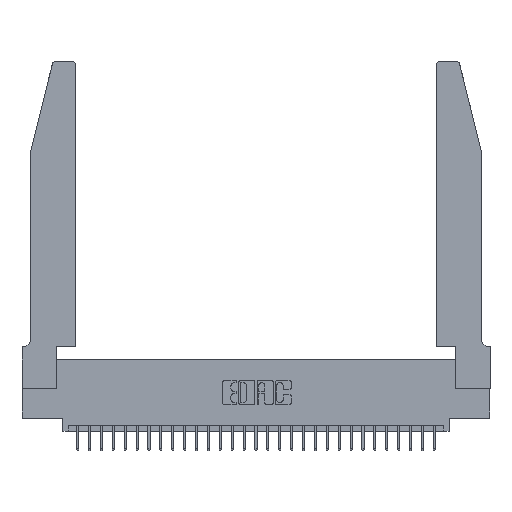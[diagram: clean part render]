
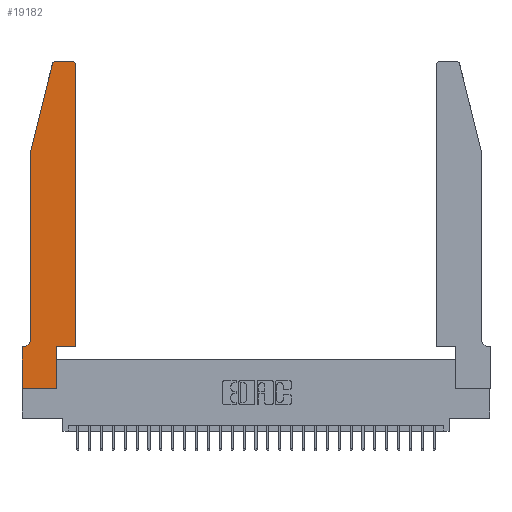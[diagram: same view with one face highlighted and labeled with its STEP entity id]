
A CAD part, top view. The second image highlights one B-rep face of the part: STEP entity #19182.
In plain terms, the highlighted planar face has unit normal (0, 0, 1).
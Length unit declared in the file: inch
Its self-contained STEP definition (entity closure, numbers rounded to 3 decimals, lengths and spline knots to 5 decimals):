
#178 = DIRECTION ( 'NONE',  ( 1., 0., 0. ) ) ;
#312 = LINE ( 'NONE', #15355, #5230 ) ;
#991 = ORIENTED_EDGE ( 'NONE', *, *, #17847, .T. ) ;
#1495 = CARTESIAN_POINT ( 'NONE',  ( 0.4505, 2.72, 0.37 ) ) ;
#1654 = CARTESIAN_POINT ( 'NONE',  ( 0.0755, 2., 0.37 ) ) ;
#1874 = CARTESIAN_POINT ( 'NONE',  ( 0.2865, 0.35, 0.37 ) ) ;
#2025 = VERTEX_POINT ( 'NONE', #1495 ) ;
#2200 = CARTESIAN_POINT ( 'NONE',  ( 0.284, 2.72, 0.37 ) ) ;
#2810 = CARTESIAN_POINT ( 'NONE',  ( 0.0755, 2., 0.37 ) ) ;
#3173 = VECTOR ( 'NONE', #6705, 39.37008 ) ;
#3685 = VECTOR ( 'NONE', #9991, 39.37008 ) ;
#4329 = ORIENTED_EDGE ( 'NONE', *, *, #30274, .T. ) ;
#4561 = CARTESIAN_POINT ( 'NONE',  ( 0.2865, 0.35, 0.37 ) ) ;
#4610 = DIRECTION ( 'NONE',  ( 1., 0., 0. ) ) ;
#4860 = VERTEX_POINT ( 'NONE', #24279 ) ;
#5037 = CARTESIAN_POINT ( 'NONE',  ( 0.4505, 0.35, 0.37 ) ) ;
#5230 = VECTOR ( 'NONE', #29594, 39.37008 ) ;
#6099 = LINE ( 'NONE', #14713, #30549 ) ;
#6434 = VECTOR ( 'NONE', #21768, 39.37008 ) ;
#6705 = DIRECTION ( 'NONE',  ( 0., 1., 0. ) ) ;
#7138 = DIRECTION ( 'NONE',  ( 0., 0., 1. ) ) ;
#7229 = VERTEX_POINT ( 'NONE', #8132 ) ;
#7371 = ORIENTED_EDGE ( 'NONE', *, *, #24773, .T. ) ;
#7495 = CARTESIAN_POINT ( 'NONE',  ( 0.2605, 2.75, 0.37 ) ) ;
#7584 = CARTESIAN_POINT ( 'NONE',  ( 0., 0., 0.37 ) ) ;
#7745 = EDGE_CURVE ( 'NONE', #14163, #13380, #26379, .T. ) ;
#7793 = CARTESIAN_POINT ( 'NONE',  ( 0., 0.35, 0.37 ) ) ;
#7902 = VECTOR ( 'NONE', #178, 39.37008 ) ;
#8132 = CARTESIAN_POINT ( 'NONE',  ( 0.0755, 2., 0.37 ) ) ;
#8502 = ORIENTED_EDGE ( 'NONE', *, *, #21854, .T. ) ;
#9805 = VERTEX_POINT ( 'NONE', #17820 ) ;
#9991 = DIRECTION ( 'NONE',  ( 1., 0., 0. ) ) ;
#10206 = DIRECTION ( 'NONE',  ( 1., 0., 0. ) ) ;
#10277 = LINE ( 'NONE', #1654, #28432 ) ;
#10327 = VERTEX_POINT ( 'NONE', #16941 ) ;
#10358 = EDGE_CURVE ( 'NONE', #25452, #18790, #20582, .T. ) ;
#10632 = DIRECTION ( 'NONE',  ( 0., 0., -1. ) ) ;
#10787 = LINE ( 'NONE', #7584, #3685 ) ;
#10956 = EDGE_CURVE ( 'NONE', #4860, #7229, #28655, .T. ) ;
#12542 = CARTESIAN_POINT ( 'NONE',  ( 0.2865, 0., 0.37 ) ) ;
#12802 = LINE ( 'NONE', #7495, #6434 ) ;
#13380 = VERTEX_POINT ( 'NONE', #18164 ) ;
#13464 = CARTESIAN_POINT ( 'NONE',  ( 0.4505, 0.35, 0.37 ) ) ;
#13768 = CIRCLE ( 'NONE', #21373, 0.03 ) ;
#14163 = VERTEX_POINT ( 'NONE', #16574 ) ;
#14263 = AXIS2_PLACEMENT_3D ( 'NONE', #24843, #10632, #27224 ) ;
#14713 = CARTESIAN_POINT ( 'NONE',  ( 0.0755, 0.35, 0.37 ) ) ;
#14776 = EDGE_CURVE ( 'NONE', #24351, #4860, #28100, .T. ) ;
#15027 = CARTESIAN_POINT ( 'NONE',  ( 0., 0.35, 0.37 ) ) ;
#15355 = CARTESIAN_POINT ( 'NONE',  ( 0., 0., 0.37 ) ) ;
#16107 = DIRECTION ( 'NONE',  ( 0., -1., 0. ) ) ;
#16574 = CARTESIAN_POINT ( 'NONE',  ( 0.0755, 0.42, 0.37 ) ) ;
#16941 = CARTESIAN_POINT ( 'NONE',  ( 0., 0., 0.37 ) ) ;
#17098 = DIRECTION ( 'NONE',  ( -1., 0., 0. ) ) ;
#17359 = EDGE_CURVE ( 'NONE', #30369, #10327, #312, .T. ) ;
#17457 = ORIENTED_EDGE ( 'NONE', *, *, #7745, .T. ) ;
#17577 = CARTESIAN_POINT ( 'NONE',  ( 0.4505, 0.35, 0.37 ) ) ;
#17629 = VECTOR ( 'NONE', #24807, 39.37008 ) ;
#17820 = CARTESIAN_POINT ( 'NONE',  ( 0.4205, 2.75, 0.37 ) ) ;
#17847 = EDGE_CURVE ( 'NONE', #10327, #26943, #10787, .T. ) ;
#18084 = EDGE_LOOP ( 'NONE', ( #4329, #27038, #27406, #7371, #17457, #28899, #24124, #991, #27813, #29283, #24515, #8502 ) ) ;
#18164 = CARTESIAN_POINT ( 'NONE',  ( 0.0055, 0.35, 0.37 ) ) ;
#18790 = VERTEX_POINT ( 'NONE', #13464 ) ;
#18932 = DIRECTION ( 'NONE',  ( 0., 0., 1. ) ) ;
#19182 = ADVANCED_FACE ( 'NONE', ( #20389 ), #24129, .T. ) ;
#19776 = AXIS2_PLACEMENT_3D ( 'NONE', #7793, #24444, #10206 ) ;
#20389 = FACE_OUTER_BOUND ( 'NONE', #18084, .T. ) ;
#20582 = LINE ( 'NONE', #5037, #7902 ) ;
#20944 = AXIS2_PLACEMENT_3D ( 'NONE', #2200, #18932, #4610 ) ;
#21373 = AXIS2_PLACEMENT_3D ( 'NONE', #21400, #7138, #23750 ) ;
#21400 = CARTESIAN_POINT ( 'NONE',  ( 0.4205, 2.72, 0.37 ) ) ;
#21768 = DIRECTION ( 'NONE',  ( -1., 0., 0. ) ) ;
#21854 = EDGE_CURVE ( 'NONE', #2025, #9805, #13768, .T. ) ;
#22399 = VECTOR ( 'NONE', #24263, 39.37008 ) ;
#23645 = LINE ( 'NONE', #1874, #3173 ) ;
#23750 = DIRECTION ( 'NONE',  ( 1., 0., 0. ) ) ;
#24124 = ORIENTED_EDGE ( 'NONE', *, *, #17359, .T. ) ;
#24129 = PLANE ( 'NONE',  #19776 ) ;
#24263 = DIRECTION ( 'NONE',  ( -0.239, -0.971, 0. ) ) ;
#24279 = CARTESIAN_POINT ( 'NONE',  ( 0.25487, 2.72718, 0.37 ) ) ;
#24351 = VERTEX_POINT ( 'NONE', #27957 ) ;
#24444 = DIRECTION ( 'NONE',  ( 0., 0., 1. ) ) ;
#24515 = ORIENTED_EDGE ( 'NONE', *, *, #26375, .T. ) ;
#24660 = LINE ( 'NONE', #17577, #17629 ) ;
#24773 = EDGE_CURVE ( 'NONE', #7229, #14163, #10277, .T. ) ;
#24807 = DIRECTION ( 'NONE',  ( 0., 1., 0. ) ) ;
#24810 = EDGE_CURVE ( 'NONE', #26943, #25452, #23645, .T. ) ;
#24843 = CARTESIAN_POINT ( 'NONE',  ( 0.0055, 0.42, 0.37 ) ) ;
#25452 = VERTEX_POINT ( 'NONE', #4561 ) ;
#25620 = EDGE_CURVE ( 'NONE', #13380, #30369, #6099, .T. ) ;
#26375 = EDGE_CURVE ( 'NONE', #18790, #2025, #24660, .T. ) ;
#26379 = CIRCLE ( 'NONE', #14263, 0.07 ) ;
#26943 = VERTEX_POINT ( 'NONE', #12542 ) ;
#27038 = ORIENTED_EDGE ( 'NONE', *, *, #14776, .T. ) ;
#27224 = DIRECTION ( 'NONE',  ( -1., 0., 0. ) ) ;
#27406 = ORIENTED_EDGE ( 'NONE', *, *, #10956, .T. ) ;
#27813 = ORIENTED_EDGE ( 'NONE', *, *, #24810, .T. ) ;
#27957 = CARTESIAN_POINT ( 'NONE',  ( 0.284, 2.75, 0.37 ) ) ;
#28100 = CIRCLE ( 'NONE', #20944, 0.03 ) ;
#28432 = VECTOR ( 'NONE', #16107, 39.37008 ) ;
#28655 = LINE ( 'NONE', #2810, #22399 ) ;
#28899 = ORIENTED_EDGE ( 'NONE', *, *, #25620, .T. ) ;
#29283 = ORIENTED_EDGE ( 'NONE', *, *, #10358, .T. ) ;
#29594 = DIRECTION ( 'NONE',  ( 0., -1., 0. ) ) ;
#30274 = EDGE_CURVE ( 'NONE', #9805, #24351, #12802, .T. ) ;
#30369 = VERTEX_POINT ( 'NONE', #15027 ) ;
#30549 = VECTOR ( 'NONE', #17098, 39.37008 ) ;
